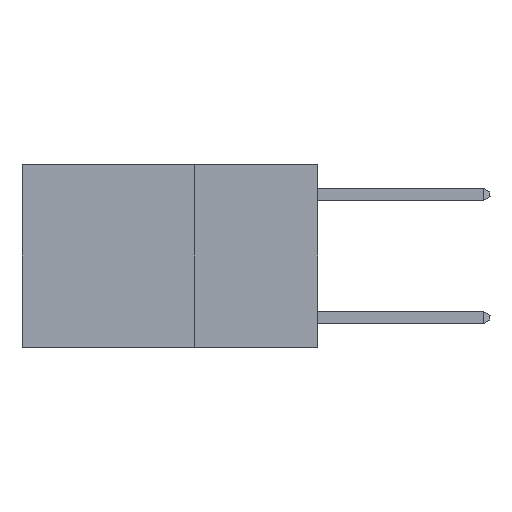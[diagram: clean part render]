
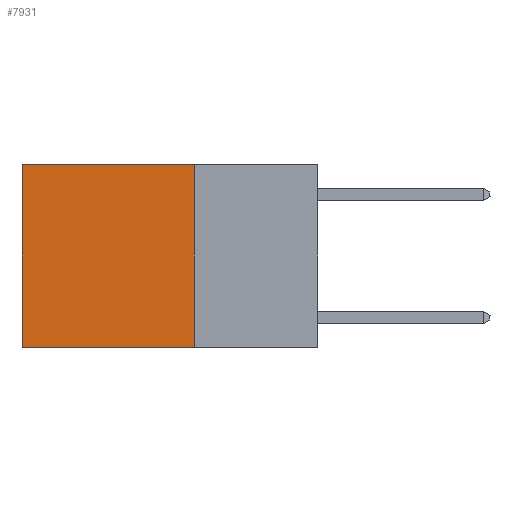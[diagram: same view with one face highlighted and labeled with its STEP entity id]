
A CAD part, left-side view. The second image highlights one B-rep face of the part: STEP entity #7931.
In plain terms, the highlighted planar face has unit normal (-1, 0, 0).
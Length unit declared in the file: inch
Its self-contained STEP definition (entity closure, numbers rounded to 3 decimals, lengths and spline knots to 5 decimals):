
#559 = VERTEX_POINT ( 'NONE', #9350 ) ;
#598 = VECTOR ( 'NONE', #13351, 39.37008 ) ;
#682 = DIRECTION ( 'NONE',  ( 0., 1., 0. ) ) ;
#818 = EDGE_CURVE ( 'NONE', #559, #12047, #8767, .T. ) ;
#824 = EDGE_CURVE ( 'NONE', #10210, #2732, #5563, .T. ) ;
#1396 = EDGE_CURVE ( 'NONE', #10210, #559, #5751, .T. ) ;
#2732 = VERTEX_POINT ( 'NONE', #5255 ) ;
#2947 = ORIENTED_EDGE ( 'NONE', *, *, #1396, .F. ) ;
#3046 = CARTESIAN_POINT ( 'NONE',  ( 0.2625, 0.6, 0. ) ) ;
#5255 = CARTESIAN_POINT ( 'NONE',  ( 0.2625, 0.6, 0. ) ) ;
#5494 = ORIENTED_EDGE ( 'NONE', *, *, #818, .F. ) ;
#5563 = LINE ( 'NONE', #12240, #11230 ) ;
#5616 = DIRECTION ( 'NONE',  ( 1., 0., 0. ) ) ;
#5623 = CARTESIAN_POINT ( 'NONE',  ( 0.2625, 0.6, -0.37 ) ) ;
#5722 = VECTOR ( 'NONE', #11933, 39.37008 ) ;
#5751 = LINE ( 'NONE', #10110, #598 ) ;
#6562 = CARTESIAN_POINT ( 'NONE',  ( 0.2625, 0.25, 0. ) ) ;
#6652 = CARTESIAN_POINT ( 'NONE',  ( 0.2625, 0.25, 0. ) ) ;
#7005 = ORIENTED_EDGE ( 'NONE', *, *, #824, .T. ) ;
#7931 = ADVANCED_FACE ( 'NONE', ( #10924 ), #12083, .F. ) ;
#8767 = LINE ( 'NONE', #12906, #13822 ) ;
#8967 = LINE ( 'NONE', #3046, #5722 ) ;
#9350 = CARTESIAN_POINT ( 'NONE',  ( 0.2625, 0.25, -0.37 ) ) ;
#10110 = CARTESIAN_POINT ( 'NONE',  ( 0.2625, 0.25, 0. ) ) ;
#10210 = VERTEX_POINT ( 'NONE', #6652 ) ;
#10924 = FACE_OUTER_BOUND ( 'NONE', #13984, .T. ) ;
#11012 = DIRECTION ( 'NONE',  ( 0., 1., 0. ) ) ;
#11230 = VECTOR ( 'NONE', #11012, 39.37008 ) ;
#11933 = DIRECTION ( 'NONE',  ( 0., 0., -1. ) ) ;
#12047 = VERTEX_POINT ( 'NONE', #5623 ) ;
#12083 = PLANE ( 'NONE',  #12534 ) ;
#12240 = CARTESIAN_POINT ( 'NONE',  ( 0.2625, 0.25, 0. ) ) ;
#12534 = AXIS2_PLACEMENT_3D ( 'NONE', #6562, #5616, #13269 ) ;
#12574 = ORIENTED_EDGE ( 'NONE', *, *, #13410, .T. ) ;
#12906 = CARTESIAN_POINT ( 'NONE',  ( 0.2625, 0.25, -0.37 ) ) ;
#13269 = DIRECTION ( 'NONE',  ( 0., 0., -1. ) ) ;
#13351 = DIRECTION ( 'NONE',  ( 0., 0., -1. ) ) ;
#13410 = EDGE_CURVE ( 'NONE', #2732, #12047, #8967, .T. ) ;
#13822 = VECTOR ( 'NONE', #682, 39.37008 ) ;
#13984 = EDGE_LOOP ( 'NONE', ( #12574, #5494, #2947, #7005 ) ) ;
